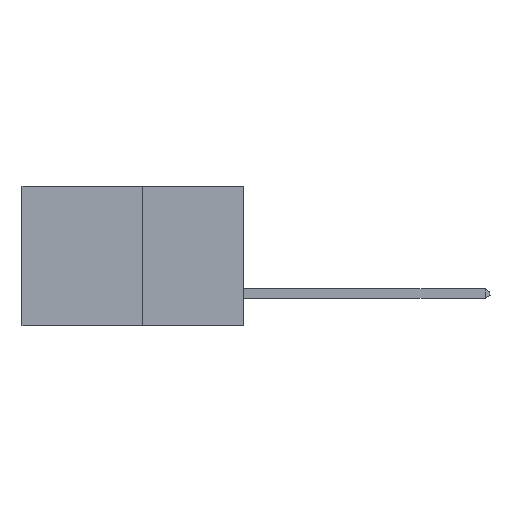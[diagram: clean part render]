
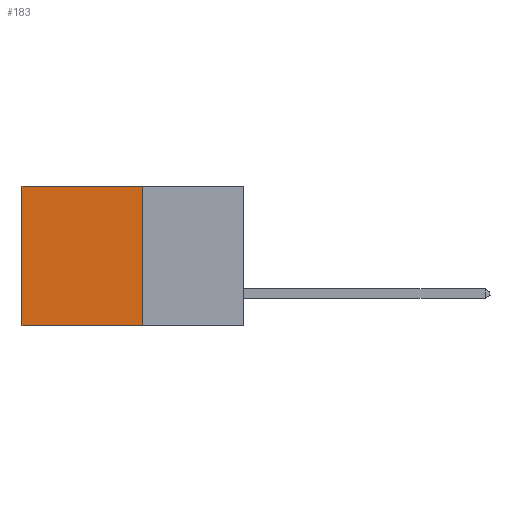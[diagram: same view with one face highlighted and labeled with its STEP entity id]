
A CAD part, left-side view. The second image highlights one B-rep face of the part: STEP entity #183.
In plain terms, the highlighted planar face has unit normal (-1, 0, 0).
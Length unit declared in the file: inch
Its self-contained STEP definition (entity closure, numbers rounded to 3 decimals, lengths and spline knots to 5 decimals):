
#183 = ADVANCED_FACE ( 'NONE', ( #4109 ), #6071, .F. ) ;
#341 = DIRECTION ( 'NONE',  ( 0., 0., -1. ) ) ;
#431 = CARTESIAN_POINT ( 'NONE',  ( 0.277, 0.59, -0.37 ) ) ;
#1882 = LINE ( 'NONE', #7325, #12151 ) ;
#1924 = ORIENTED_EDGE ( 'NONE', *, *, #11691, .T. ) ;
#3449 = DIRECTION ( 'NONE',  ( 0., 1., 0. ) ) ;
#3853 = ORIENTED_EDGE ( 'NONE', *, *, #16850, .F. ) ;
#3883 = CARTESIAN_POINT ( 'NONE',  ( 0.277, 0.27, 0. ) ) ;
#4109 = FACE_OUTER_BOUND ( 'NONE', #13171, .T. ) ;
#4639 = LINE ( 'NONE', #16009, #12079 ) ;
#5098 = DIRECTION ( 'NONE',  ( 0., 0., -1. ) ) ;
#5309 = ORIENTED_EDGE ( 'NONE', *, *, #15719, .F. ) ;
#6071 = PLANE ( 'NONE',  #13715 ) ;
#6139 = LINE ( 'NONE', #11419, #9246 ) ;
#7325 = CARTESIAN_POINT ( 'NONE',  ( 0.277, 0.27, -0.37 ) ) ;
#7543 = VERTEX_POINT ( 'NONE', #431 ) ;
#8410 = DIRECTION ( 'NONE',  ( 0., 1., 0. ) ) ;
#9150 = EDGE_CURVE ( 'NONE', #15375, #7543, #12387, .T. ) ;
#9246 = VECTOR ( 'NONE', #3449, 39.37008 ) ;
#9347 = VECTOR ( 'NONE', #5098, 39.37008 ) ;
#10454 = CARTESIAN_POINT ( 'NONE',  ( 0.277, 0.59, 0. ) ) ;
#10962 = ORIENTED_EDGE ( 'NONE', *, *, #9150, .T. ) ;
#11419 = CARTESIAN_POINT ( 'NONE',  ( 0.277, 0.27, 0. ) ) ;
#11691 = EDGE_CURVE ( 'NONE', #16630, #15375, #6139, .T. ) ;
#12079 = VECTOR ( 'NONE', #8410, 39.37008 ) ;
#12151 = VECTOR ( 'NONE', #16178, 39.37008 ) ;
#12387 = LINE ( 'NONE', #12923, #9347 ) ;
#12923 = CARTESIAN_POINT ( 'NONE',  ( 0.277, 0.59, -0.37 ) ) ;
#13171 = EDGE_LOOP ( 'NONE', ( #10962, #3853, #5309, #1924 ) ) ;
#13715 = AXIS2_PLACEMENT_3D ( 'NONE', #14277, #15972, #341 ) ;
#14277 = CARTESIAN_POINT ( 'NONE',  ( 0.277, 0.27, -0.37 ) ) ;
#14929 = VERTEX_POINT ( 'NONE', #16779 ) ;
#15375 = VERTEX_POINT ( 'NONE', #10454 ) ;
#15719 = EDGE_CURVE ( 'NONE', #16630, #14929, #1882, .T. ) ;
#15972 = DIRECTION ( 'NONE',  ( 1., 0., 0. ) ) ;
#16009 = CARTESIAN_POINT ( 'NONE',  ( 0.277, 0.27, -0.37 ) ) ;
#16178 = DIRECTION ( 'NONE',  ( 0., 0., -1. ) ) ;
#16630 = VERTEX_POINT ( 'NONE', #3883 ) ;
#16779 = CARTESIAN_POINT ( 'NONE',  ( 0.277, 0.27, -0.37 ) ) ;
#16850 = EDGE_CURVE ( 'NONE', #14929, #7543, #4639, .T. ) ;
